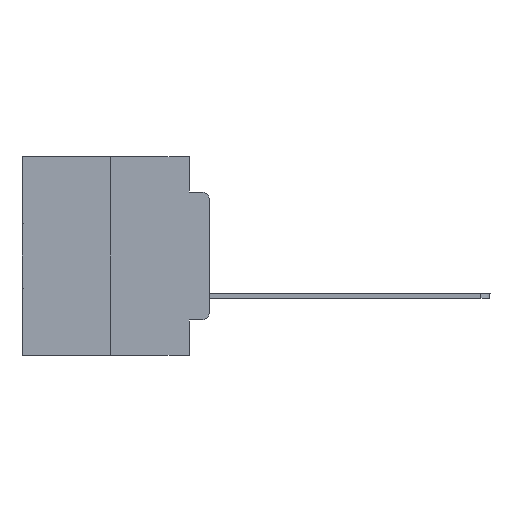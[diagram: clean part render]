
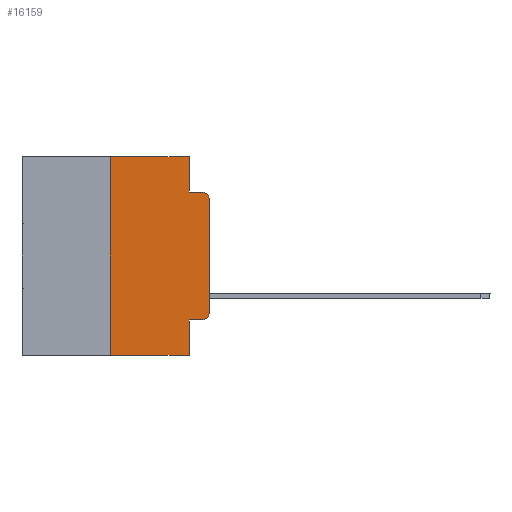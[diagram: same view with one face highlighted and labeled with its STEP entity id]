
A CAD part, left-side view. The second image highlights one B-rep face of the part: STEP entity #16159.
In plain terms, the highlighted planar face has unit normal (-1, 0, 0).
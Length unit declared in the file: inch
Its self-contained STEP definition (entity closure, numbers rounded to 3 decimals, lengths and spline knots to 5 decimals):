
#579 = AXIS2_PLACEMENT_3D ( 'NONE', #13833, #11363, #26028 ) ;
#1164 = VERTEX_POINT ( 'NONE', #2896 ) ;
#1285 = EDGE_CURVE ( 'NONE', #9293, #6495, #29462, .T. ) ;
#1593 = CARTESIAN_POINT ( 'NONE',  ( 0., 0.051, 0. ) ) ;
#1612 = EDGE_CURVE ( 'NONE', #29007, #9293, #21169, .T. ) ;
#1752 = LINE ( 'NONE', #1593, #27022 ) ;
#1828 = ORIENTED_EDGE ( 'NONE', *, *, #30315, .T. ) ;
#2364 = DIRECTION ( 'NONE',  ( 1., 0., 0. ) ) ;
#2429 = VERTEX_POINT ( 'NONE', #29955 ) ;
#2896 = CARTESIAN_POINT ( 'NONE',  ( 0., 0.25, -0.5 ) ) ;
#2916 = ORIENTED_EDGE ( 'NONE', *, *, #7413, .T. ) ;
#3271 = VERTEX_POINT ( 'NONE', #5476 ) ;
#4573 = ORIENTED_EDGE ( 'NONE', *, *, #26404, .F. ) ;
#4817 = CARTESIAN_POINT ( 'NONE',  ( 0., 0.051, -0.0885 ) ) ;
#4878 = DIRECTION ( 'NONE',  ( -1., 0., 0. ) ) ;
#4883 = VECTOR ( 'NONE', #24209, 39.37008 ) ;
#5476 = CARTESIAN_POINT ( 'NONE',  ( 0., 0.051, -0.5 ) ) ;
#6419 = VERTEX_POINT ( 'NONE', #16129 ) ;
#6495 = VERTEX_POINT ( 'NONE', #11327 ) ;
#6818 = LINE ( 'NONE', #27820, #16644 ) ;
#6838 = ORIENTED_EDGE ( 'NONE', *, *, #13789, .F. ) ;
#7037 = CARTESIAN_POINT ( 'NONE',  ( 0., 0.02, -0.3915 ) ) ;
#7413 = EDGE_CURVE ( 'NONE', #6495, #7552, #16909, .T. ) ;
#7552 = VERTEX_POINT ( 'NONE', #14609 ) ;
#7887 = LINE ( 'NONE', #28663, #26181 ) ;
#8197 = VERTEX_POINT ( 'NONE', #27654 ) ;
#9293 = VERTEX_POINT ( 'NONE', #20584 ) ;
#9834 = AXIS2_PLACEMENT_3D ( 'NONE', #7037, #4878, #23434 ) ;
#10566 = VECTOR ( 'NONE', #24121, 39.37008 ) ;
#11327 = CARTESIAN_POINT ( 'NONE',  ( 0., 0., -0.1085 ) ) ;
#11363 = DIRECTION ( 'NONE',  ( -1., 0., 0. ) ) ;
#11375 = DIRECTION ( 'NONE',  ( 0., -1., 0. ) ) ;
#12363 = EDGE_CURVE ( 'NONE', #1164, #2429, #13777, .T. ) ;
#12771 = ORIENTED_EDGE ( 'NONE', *, *, #1285, .T. ) ;
#13257 = CARTESIAN_POINT ( 'NONE',  ( 0., 0.051, -0.4115 ) ) ;
#13379 = ORIENTED_EDGE ( 'NONE', *, *, #12363, .F. ) ;
#13709 = LINE ( 'NONE', #13257, #15183 ) ;
#13777 = LINE ( 'NONE', #30006, #16417 ) ;
#13789 = EDGE_CURVE ( 'NONE', #8197, #7552, #26266, .T. ) ;
#13804 = DIRECTION ( 'NONE',  ( 0., 0., -1. ) ) ;
#13833 = CARTESIAN_POINT ( 'NONE',  ( 0., 0.02, -0.1085 ) ) ;
#13927 = DIRECTION ( 'NONE',  ( 0., 0., 1. ) ) ;
#14383 = CARTESIAN_POINT ( 'NONE',  ( 0., 0.02, -0.4115 ) ) ;
#14609 = CARTESIAN_POINT ( 'NONE',  ( 0., 0.02, -0.0885 ) ) ;
#15183 = VECTOR ( 'NONE', #11375, 39.37008 ) ;
#15751 = VERTEX_POINT ( 'NONE', #21105 ) ;
#16099 = DIRECTION ( 'NONE',  ( 0., -1., 0. ) ) ;
#16129 = CARTESIAN_POINT ( 'NONE',  ( 0., 0.051, -0.4115 ) ) ;
#16159 = ADVANCED_FACE ( 'NONE', ( #21070 ), #30179, .F. ) ;
#16404 = DIRECTION ( 'NONE',  ( 0., 0., -1. ) ) ;
#16417 = VECTOR ( 'NONE', #13927, 39.37008 ) ;
#16644 = VECTOR ( 'NONE', #16099, 39.37008 ) ;
#16909 = CIRCLE ( 'NONE', #579, 0.02 ) ;
#17403 = DIRECTION ( 'NONE',  ( 0., -1., 0. ) ) ;
#17770 = EDGE_CURVE ( 'NONE', #6419, #3271, #20880, .T. ) ;
#18464 = CARTESIAN_POINT ( 'NONE',  ( 0., 0.473, 0. ) ) ;
#19960 = AXIS2_PLACEMENT_3D ( 'NONE', #18464, #2364, #13804 ) ;
#19974 = ORIENTED_EDGE ( 'NONE', *, *, #1612, .T. ) ;
#20584 = CARTESIAN_POINT ( 'NONE',  ( 0., 0., -0.3915 ) ) ;
#20587 = CARTESIAN_POINT ( 'NONE',  ( 0., 0.051, 0. ) ) ;
#20880 = LINE ( 'NONE', #20587, #28132 ) ;
#21070 = FACE_OUTER_BOUND ( 'NONE', #26320, .T. ) ;
#21105 = CARTESIAN_POINT ( 'NONE',  ( 0., 0.051, 0. ) ) ;
#21169 = CIRCLE ( 'NONE', #9834, 0.02 ) ;
#23434 = DIRECTION ( 'NONE',  ( 0., 0., -1. ) ) ;
#24121 = DIRECTION ( 'NONE',  ( 0., -1., 0. ) ) ;
#24209 = DIRECTION ( 'NONE',  ( 0., 0., 1. ) ) ;
#24225 = ORIENTED_EDGE ( 'NONE', *, *, #26849, .T. ) ;
#25395 = DIRECTION ( 'NONE',  ( 0., 0., -1. ) ) ;
#26028 = DIRECTION ( 'NONE',  ( 0., 0., -1. ) ) ;
#26181 = VECTOR ( 'NONE', #17403, 39.37008 ) ;
#26266 = LINE ( 'NONE', #4817, #10566 ) ;
#26320 = EDGE_LOOP ( 'NONE', ( #12771, #2916, #6838, #28217, #4573, #13379, #1828, #29019, #24225, #19974 ) ) ;
#26404 = EDGE_CURVE ( 'NONE', #2429, #15751, #6818, .T. ) ;
#26849 = EDGE_CURVE ( 'NONE', #6419, #29007, #13709, .T. ) ;
#27022 = VECTOR ( 'NONE', #25395, 39.37008 ) ;
#27252 = EDGE_CURVE ( 'NONE', #15751, #8197, #1752, .T. ) ;
#27654 = CARTESIAN_POINT ( 'NONE',  ( 0., 0.051, -0.0885 ) ) ;
#27820 = CARTESIAN_POINT ( 'NONE',  ( 0., 0.473, 0. ) ) ;
#28132 = VECTOR ( 'NONE', #16404, 39.37008 ) ;
#28217 = ORIENTED_EDGE ( 'NONE', *, *, #27252, .F. ) ;
#28663 = CARTESIAN_POINT ( 'NONE',  ( 0., 0.473, -0.5 ) ) ;
#29007 = VERTEX_POINT ( 'NONE', #14383 ) ;
#29019 = ORIENTED_EDGE ( 'NONE', *, *, #17770, .F. ) ;
#29311 = CARTESIAN_POINT ( 'NONE',  ( 0., 0., 0. ) ) ;
#29462 = LINE ( 'NONE', #29311, #4883 ) ;
#29955 = CARTESIAN_POINT ( 'NONE',  ( 0., 0.25, 0. ) ) ;
#30006 = CARTESIAN_POINT ( 'NONE',  ( 0., 0.25, 0. ) ) ;
#30179 = PLANE ( 'NONE',  #19960 ) ;
#30315 = EDGE_CURVE ( 'NONE', #1164, #3271, #7887, .T. ) ;
